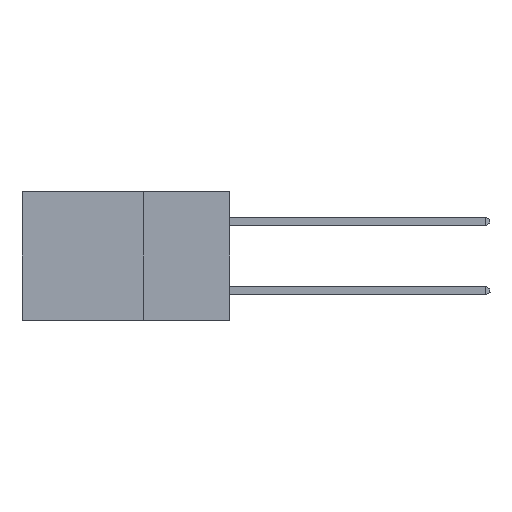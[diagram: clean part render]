
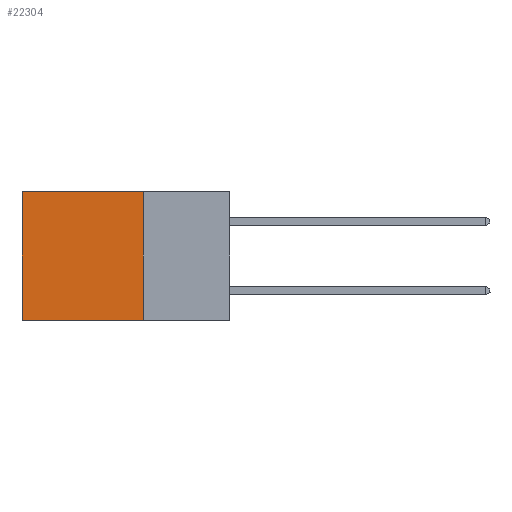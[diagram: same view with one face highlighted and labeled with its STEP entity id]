
A CAD part, left-side view. The second image highlights one B-rep face of the part: STEP entity #22304.
In plain terms, the highlighted planar face has unit normal (-1, 0, 0).
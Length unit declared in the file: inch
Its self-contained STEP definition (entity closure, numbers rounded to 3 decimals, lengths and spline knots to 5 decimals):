
#97 = DIRECTION ( 'NONE',  ( 0., 0., -1. ) ) ;
#890 = VERTEX_POINT ( 'NONE', #23019 ) ;
#1500 = PLANE ( 'NONE',  #15721 ) ;
#1696 = VERTEX_POINT ( 'NONE', #5343 ) ;
#2079 = ORIENTED_EDGE ( 'NONE', *, *, #25771, .F. ) ;
#2194 = CARTESIAN_POINT ( 'NONE',  ( 0.298, 0.25, 0. ) ) ;
#2816 = CARTESIAN_POINT ( 'NONE',  ( 0.298, 0.6, 0. ) ) ;
#2990 = LINE ( 'NONE', #19852, #13181 ) ;
#3259 = VERTEX_POINT ( 'NONE', #2816 ) ;
#3474 = ORIENTED_EDGE ( 'NONE', *, *, #4752, .T. ) ;
#3574 = CARTESIAN_POINT ( 'NONE',  ( 0.298, 0.25, 0. ) ) ;
#4752 = EDGE_CURVE ( 'NONE', #890, #3259, #11714, .T. ) ;
#5084 = ORIENTED_EDGE ( 'NONE', *, *, #24281, .F. ) ;
#5343 = CARTESIAN_POINT ( 'NONE',  ( 0.298, 0.6, -0.37 ) ) ;
#6131 = VECTOR ( 'NONE', #21187, 39.37008 ) ;
#6772 = LINE ( 'NONE', #15227, #6131 ) ;
#7341 = ORIENTED_EDGE ( 'NONE', *, *, #25412, .T. ) ;
#7540 = FACE_OUTER_BOUND ( 'NONE', #8386, .T. ) ;
#7681 = DIRECTION ( 'NONE',  ( 0., 0., -1. ) ) ;
#7846 = VERTEX_POINT ( 'NONE', #23558 ) ;
#8386 = EDGE_LOOP ( 'NONE', ( #7341, #5084, #2079, #3474 ) ) ;
#10960 = CARTESIAN_POINT ( 'NONE',  ( 0.298, 0.25, 0. ) ) ;
#11714 = LINE ( 'NONE', #10960, #20967 ) ;
#12987 = DIRECTION ( 'NONE',  ( 0., 1., 0. ) ) ;
#13181 = VECTOR ( 'NONE', #15987, 39.37008 ) ;
#15227 = CARTESIAN_POINT ( 'NONE',  ( 0.298, 0.6, 0. ) ) ;
#15721 = AXIS2_PLACEMENT_3D ( 'NONE', #3574, #19667, #7681 ) ;
#15987 = DIRECTION ( 'NONE',  ( 0., 1., 0. ) ) ;
#19667 = DIRECTION ( 'NONE',  ( 1., 0., 0. ) ) ;
#19852 = CARTESIAN_POINT ( 'NONE',  ( 0.298, 0.25, -0.37 ) ) ;
#20967 = VECTOR ( 'NONE', #12987, 39.37008 ) ;
#21187 = DIRECTION ( 'NONE',  ( 0., 0., -1. ) ) ;
#22304 = ADVANCED_FACE ( 'NONE', ( #7540 ), #1500, .F. ) ;
#23019 = CARTESIAN_POINT ( 'NONE',  ( 0.298, 0.25, 0. ) ) ;
#23297 = VECTOR ( 'NONE', #97, 39.37008 ) ;
#23558 = CARTESIAN_POINT ( 'NONE',  ( 0.298, 0.25, -0.37 ) ) ;
#23925 = LINE ( 'NONE', #2194, #23297 ) ;
#24281 = EDGE_CURVE ( 'NONE', #7846, #1696, #2990, .T. ) ;
#25412 = EDGE_CURVE ( 'NONE', #3259, #1696, #6772, .T. ) ;
#25771 = EDGE_CURVE ( 'NONE', #890, #7846, #23925, .T. ) ;
